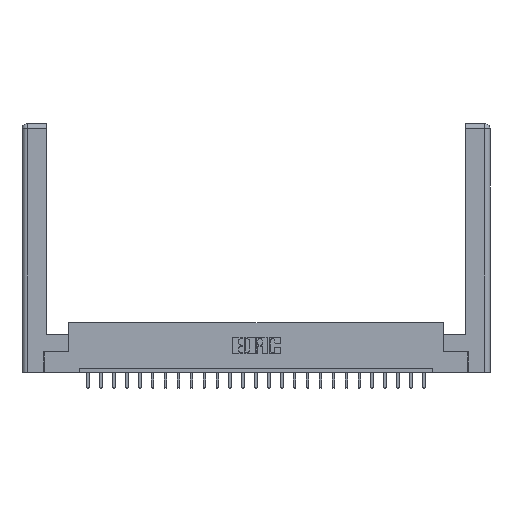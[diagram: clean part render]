
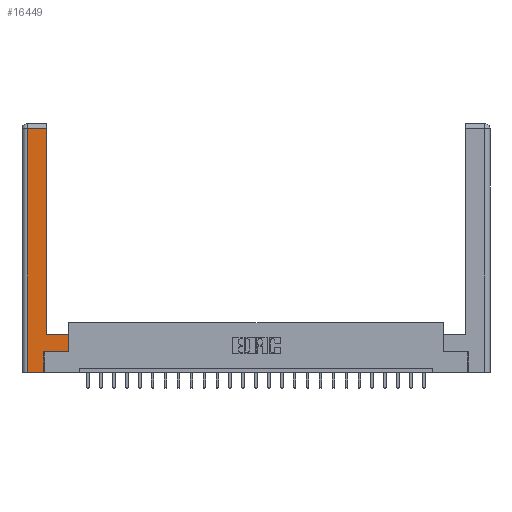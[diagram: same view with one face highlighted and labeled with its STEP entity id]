
A CAD part, top view. The second image highlights one B-rep face of the part: STEP entity #16449.
In plain terms, the highlighted planar face has unit normal (0, 0, 1).
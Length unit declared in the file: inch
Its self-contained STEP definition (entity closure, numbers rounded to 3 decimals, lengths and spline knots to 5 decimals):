
#579 = DIRECTION ( 'NONE',  ( 0., -1., 0. ) ) ;
#697 = DIRECTION ( 'NONE',  ( 0., 1., 0. ) ) ;
#1028 = EDGE_LOOP ( 'NONE', ( #22818, #14165, #9411, #3656, #19982, #21184, #20691, #24031 ) ) ;
#1353 = VECTOR ( 'NONE', #697, 39.37008 ) ;
#1512 = DIRECTION ( 'NONE',  ( -1., 0., 0. ) ) ;
#1727 = EDGE_CURVE ( 'NONE', #23571, #3213, #14484, .T. ) ;
#2715 = CARTESIAN_POINT ( 'NONE',  ( 0.0615, 0., 0. ) ) ;
#3213 = VERTEX_POINT ( 'NONE', #17730 ) ;
#3360 = AXIS2_PLACEMENT_3D ( 'NONE', #15013, #17029, #1512 ) ;
#3523 = DIRECTION ( 'NONE',  ( 0., 1., 0. ) ) ;
#3656 = ORIENTED_EDGE ( 'NONE', *, *, #17340, .T. ) ;
#3964 = CARTESIAN_POINT ( 'NONE',  ( 0.565, 0.45, 0. ) ) ;
#5986 = FACE_OUTER_BOUND ( 'NONE', #1028, .T. ) ;
#6152 = CARTESIAN_POINT ( 'NONE',  ( 0.565, 0.245, 0. ) ) ;
#6865 = CARTESIAN_POINT ( 'NONE',  ( 0.565, 0.45, 0. ) ) ;
#7263 = VECTOR ( 'NONE', #19241, 39.37008 ) ;
#7291 = VERTEX_POINT ( 'NONE', #11433 ) ;
#7427 = LINE ( 'NONE', #6152, #11262 ) ;
#7677 = LINE ( 'NONE', #13474, #20190 ) ;
#7801 = EDGE_CURVE ( 'NONE', #8805, #10214, #7427, .T. ) ;
#8501 = EDGE_CURVE ( 'NONE', #7291, #18068, #7677, .T. ) ;
#8805 = VERTEX_POINT ( 'NONE', #16099 ) ;
#8839 = VECTOR ( 'NONE', #10242, 39.37008 ) ;
#9209 = LINE ( 'NONE', #17100, #13997 ) ;
#9411 = ORIENTED_EDGE ( 'NONE', *, *, #20265, .T. ) ;
#9492 = LINE ( 'NONE', #22991, #11583 ) ;
#9726 = CARTESIAN_POINT ( 'NONE',  ( 0.0615, 2.94, 0. ) ) ;
#10214 = VERTEX_POINT ( 'NONE', #20791 ) ;
#10242 = DIRECTION ( 'NONE',  ( -1., 0., 0. ) ) ;
#11262 = VECTOR ( 'NONE', #19580, 39.37008 ) ;
#11265 = DIRECTION ( 'NONE',  ( 1., 0., 0. ) ) ;
#11433 = CARTESIAN_POINT ( 'NONE',  ( 0.295, 2.94, 0. ) ) ;
#11583 = VECTOR ( 'NONE', #579, 39.37008 ) ;
#12071 = CARTESIAN_POINT ( 'NONE',  ( 0.295, 0.45, 0. ) ) ;
#12125 = CARTESIAN_POINT ( 'NONE',  ( 0.265, 0.245, 0. ) ) ;
#13263 = VERTEX_POINT ( 'NONE', #18997 ) ;
#13474 = CARTESIAN_POINT ( 'NONE',  ( 0.0615, 2.94, 0. ) ) ;
#13745 = EDGE_CURVE ( 'NONE', #13263, #8805, #21696, .T. ) ;
#13997 = VECTOR ( 'NONE', #3523, 39.37008 ) ;
#14165 = ORIENTED_EDGE ( 'NONE', *, *, #8501, .T. ) ;
#14484 = LINE ( 'NONE', #12071, #8839 ) ;
#15013 = CARTESIAN_POINT ( 'NONE',  ( 0., 0., 0. ) ) ;
#15373 = DIRECTION ( 'NONE',  ( -1., 0., 0. ) ) ;
#15769 = VECTOR ( 'NONE', #11265, 39.37008 ) ;
#16099 = CARTESIAN_POINT ( 'NONE',  ( 0.265, 0.245, 0. ) ) ;
#16449 = ADVANCED_FACE ( 'NONE', ( #5986 ), #22567, .F. ) ;
#17029 = DIRECTION ( 'NONE',  ( 0., 0., -1. ) ) ;
#17100 = CARTESIAN_POINT ( 'NONE',  ( 0.295, 3., 0. ) ) ;
#17340 = EDGE_CURVE ( 'NONE', #21704, #13263, #20890, .T. ) ;
#17372 = EDGE_CURVE ( 'NONE', #3213, #7291, #9209, .T. ) ;
#17730 = CARTESIAN_POINT ( 'NONE',  ( 0.295, 0.45, 0. ) ) ;
#18068 = VERTEX_POINT ( 'NONE', #9726 ) ;
#18997 = CARTESIAN_POINT ( 'NONE',  ( 0.265, 0., 0. ) ) ;
#19241 = DIRECTION ( 'NONE',  ( 0., 1., 0. ) ) ;
#19580 = DIRECTION ( 'NONE',  ( 1., 0., 0. ) ) ;
#19982 = ORIENTED_EDGE ( 'NONE', *, *, #13745, .T. ) ;
#20190 = VECTOR ( 'NONE', #15373, 39.37008 ) ;
#20265 = EDGE_CURVE ( 'NONE', #18068, #21704, #9492, .T. ) ;
#20691 = ORIENTED_EDGE ( 'NONE', *, *, #23086, .T. ) ;
#20791 = CARTESIAN_POINT ( 'NONE',  ( 0.565, 0.245, 0. ) ) ;
#20890 = LINE ( 'NONE', #22828, #15769 ) ;
#21184 = ORIENTED_EDGE ( 'NONE', *, *, #7801, .T. ) ;
#21696 = LINE ( 'NONE', #12125, #1353 ) ;
#21704 = VERTEX_POINT ( 'NONE', #2715 ) ;
#22485 = LINE ( 'NONE', #3964, #7263 ) ;
#22567 = PLANE ( 'NONE',  #3360 ) ;
#22818 = ORIENTED_EDGE ( 'NONE', *, *, #17372, .T. ) ;
#22828 = CARTESIAN_POINT ( 'NONE',  ( 0.265, 0., 0. ) ) ;
#22991 = CARTESIAN_POINT ( 'NONE',  ( 0.0615, 0., 0. ) ) ;
#23086 = EDGE_CURVE ( 'NONE', #10214, #23571, #22485, .T. ) ;
#23571 = VERTEX_POINT ( 'NONE', #6865 ) ;
#24031 = ORIENTED_EDGE ( 'NONE', *, *, #1727, .T. ) ;
